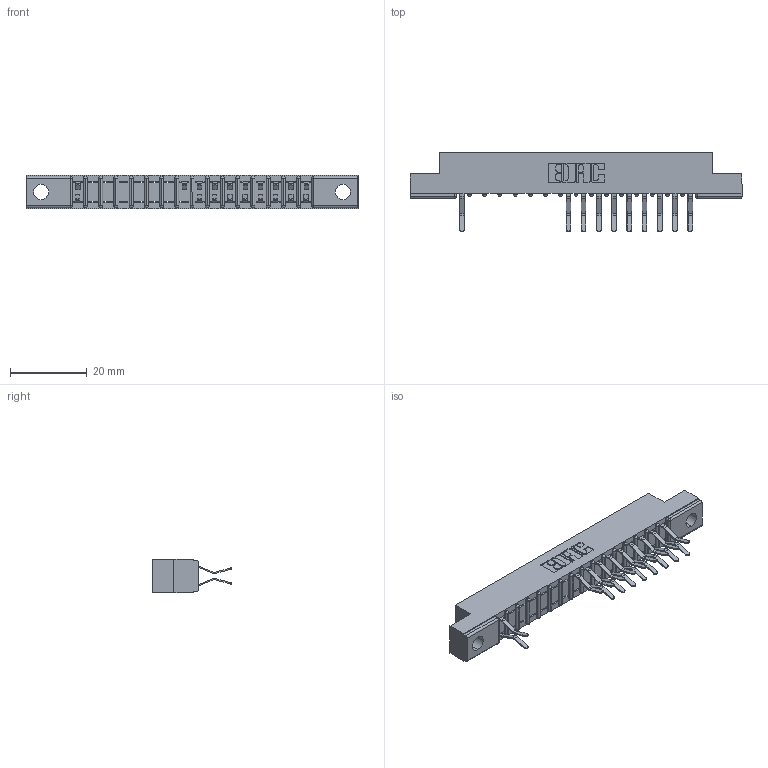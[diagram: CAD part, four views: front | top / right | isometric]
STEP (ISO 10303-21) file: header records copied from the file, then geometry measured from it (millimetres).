
FILE_DESCRIPTION (( 'STEP AP203' ), '1' );
FILE_NAME ('307-032-560-204.STEP', '2018-08-04T23:00:54', ( '' ), ( '' ), 'SwSTEP 2.0', 'SolidWorks 2016', '' );
FILE_SCHEMA (( 'CONFIG_CONTROL_DESIGN' ));
Length unit declared in the file: inch
Products named in the file (3): 307 Part_.156 Dia Mounting Holes; 307-290-001_560; 307-032-560-204
Assembly tree (20 placements, depth 2):
  307-032-560-204
    307 Part_.156 Dia Mounting Holes
    307-290-001_560  x19
Bounding box: 86.41 x 20.73 x 8.71 mm (x, y, z)
Volume: 5402.3 mm3; surface area: 8267.2 mm2
Topology: 20 solids, 20 shells, 1229 faces, 3473 edges, 2242 vertices
Faces by surface type: plane 789, cylinder 406, sphere 34
Entity records: 17540 total; most frequent: CARTESIAN_POINT 2937, ORIENTED_EDGE 2918, DIRECTION 2867, EDGE_CURVE 1459, VECTOR 1115, LINE 1115, VERTEX_POINT 946, AXIS2_PLACEMENT_3D 876
